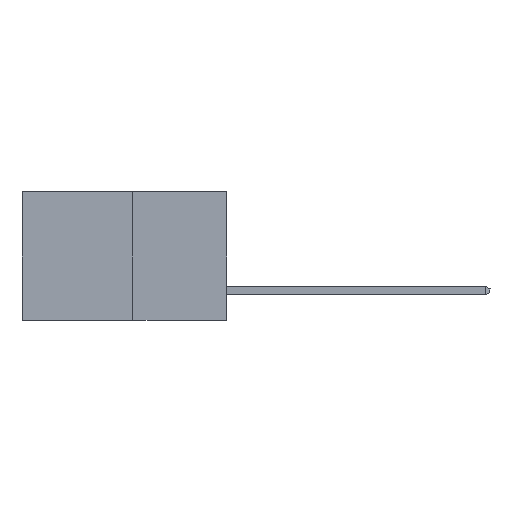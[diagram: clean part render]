
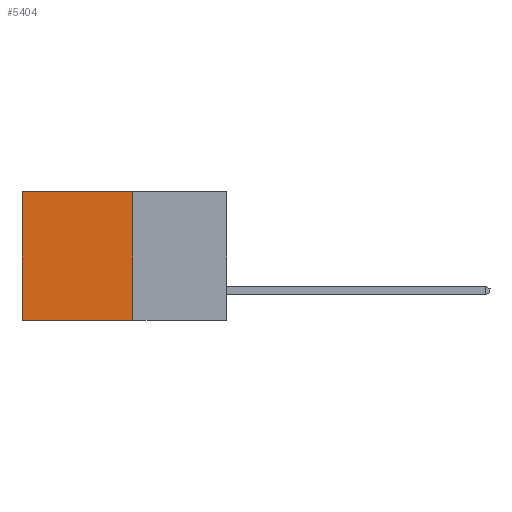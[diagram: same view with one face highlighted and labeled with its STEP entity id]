
A CAD part, left-side view. The second image highlights one B-rep face of the part: STEP entity #5404.
In plain terms, the highlighted planar face has unit normal (-1, 0, 0).
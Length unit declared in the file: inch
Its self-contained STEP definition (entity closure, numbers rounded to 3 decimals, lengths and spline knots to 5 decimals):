
#21 = LINE ( 'NONE', #12564, #12157 ) ;
#385 = CARTESIAN_POINT ( 'NONE',  ( 0.277, 0.27, 0. ) ) ;
#1122 = CARTESIAN_POINT ( 'NONE',  ( 0.277, 0.59, -0.37 ) ) ;
#1637 = VECTOR ( 'NONE', #3451, 39.37008 ) ;
#1898 = VERTEX_POINT ( 'NONE', #385 ) ;
#2227 = CARTESIAN_POINT ( 'NONE',  ( 0.277, 0.27, -0.37 ) ) ;
#2288 = DIRECTION ( 'NONE',  ( 0., 1., 0. ) ) ;
#2923 = VERTEX_POINT ( 'NONE', #8018 ) ;
#3174 = EDGE_CURVE ( 'NONE', #2923, #13286, #6798, .T. ) ;
#3349 = DIRECTION ( 'NONE',  ( 0., 0., -1. ) ) ;
#3451 = DIRECTION ( 'NONE',  ( 0., 0., -1. ) ) ;
#3809 = VERTEX_POINT ( 'NONE', #5127 ) ;
#3836 = DIRECTION ( 'NONE',  ( 0., 1., 0. ) ) ;
#4135 = EDGE_CURVE ( 'NONE', #1898, #3809, #21, .T. ) ;
#4649 = LINE ( 'NONE', #11471, #1637 ) ;
#5127 = CARTESIAN_POINT ( 'NONE',  ( 0.277, 0.59, 0. ) ) ;
#5404 = ADVANCED_FACE ( 'NONE', ( #10171 ), #10562, .F. ) ;
#5997 = DIRECTION ( 'NONE',  ( 0., 0., -1. ) ) ;
#6798 = LINE ( 'NONE', #7275, #10243 ) ;
#7275 = CARTESIAN_POINT ( 'NONE',  ( 0.277, 0.27, -0.37 ) ) ;
#7788 = LINE ( 'NONE', #2227, #10835 ) ;
#8018 = CARTESIAN_POINT ( 'NONE',  ( 0.277, 0.27, -0.37 ) ) ;
#8802 = EDGE_LOOP ( 'NONE', ( #13658, #11379, #12088, #12781 ) ) ;
#9085 = EDGE_CURVE ( 'NONE', #1898, #2923, #7788, .T. ) ;
#10171 = FACE_OUTER_BOUND ( 'NONE', #8802, .T. ) ;
#10243 = VECTOR ( 'NONE', #3836, 39.37008 ) ;
#10255 = AXIS2_PLACEMENT_3D ( 'NONE', #11707, #12823, #5997 ) ;
#10562 = PLANE ( 'NONE',  #10255 ) ;
#10835 = VECTOR ( 'NONE', #3349, 39.37008 ) ;
#11379 = ORIENTED_EDGE ( 'NONE', *, *, #3174, .F. ) ;
#11471 = CARTESIAN_POINT ( 'NONE',  ( 0.277, 0.59, -0.37 ) ) ;
#11707 = CARTESIAN_POINT ( 'NONE',  ( 0.277, 0.27, -0.37 ) ) ;
#12088 = ORIENTED_EDGE ( 'NONE', *, *, #9085, .F. ) ;
#12157 = VECTOR ( 'NONE', #2288, 39.37008 ) ;
#12564 = CARTESIAN_POINT ( 'NONE',  ( 0.277, 0.27, 0. ) ) ;
#12698 = EDGE_CURVE ( 'NONE', #3809, #13286, #4649, .T. ) ;
#12781 = ORIENTED_EDGE ( 'NONE', *, *, #4135, .T. ) ;
#12823 = DIRECTION ( 'NONE',  ( 1., 0., 0. ) ) ;
#13286 = VERTEX_POINT ( 'NONE', #1122 ) ;
#13658 = ORIENTED_EDGE ( 'NONE', *, *, #12698, .T. ) ;
